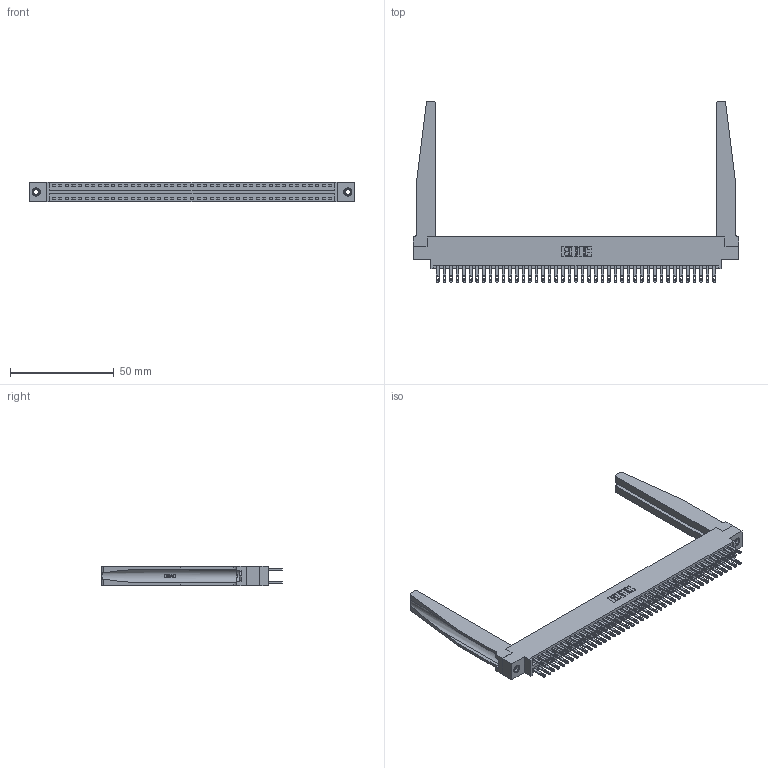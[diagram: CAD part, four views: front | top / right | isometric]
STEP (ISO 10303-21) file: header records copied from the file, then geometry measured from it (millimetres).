
FILE_DESCRIPTION (( 'STEP AP203' ), '1' );
FILE_NAME ('346-086-500-878.STEP', '2022-05-25T21:35:43', ( '' ), ( '' ), 'SwSTEP 2.0', 'SolidWorks 2020', '' );
FILE_SCHEMA (( 'CONFIG_CONTROL_DESIGN' ));
Length unit declared in the file: inch
Products named in the file (5): 345-250-001_345-250-001-102; 346-220-078_345-220-078; 346 Part_0.170 Offset - 0.156 Dia-TH; 346-086-500-878; 345-292-001_345-293-100
Assembly tree (91 placements, depth 2):
  346-086-500-878
    346 Part_0.170 Offset - 0.156 Dia-TH
    345-292-001_345-293-100  x86
    346-220-078_345-220-078  x2
    345-250-001_345-250-001-102  x2
Bounding box: 157.1 x 87.12 x 9.4 mm (x, y, z)
Volume: 22325.8 mm3; surface area: 28859.2 mm2
Topology: 91 solids, 91 shells, 4502 faces, 13627 edges, 9074 vertices
Faces by surface type: plane 2730, cylinder 1720, bspline 36, cone 12, torus 4
Entity records: 33154 total; most frequent: CARTESIAN_POINT 6405, ORIENTED_EDGE 5226, DIRECTION 4683, EDGE_CURVE 2613, LINE 2211, VECTOR 2211, VERTEX_POINT 1736, AXIS2_PLACEMENT_3D 1236
